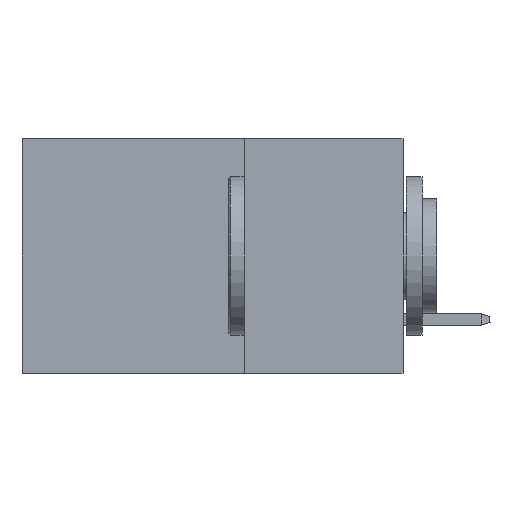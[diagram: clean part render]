
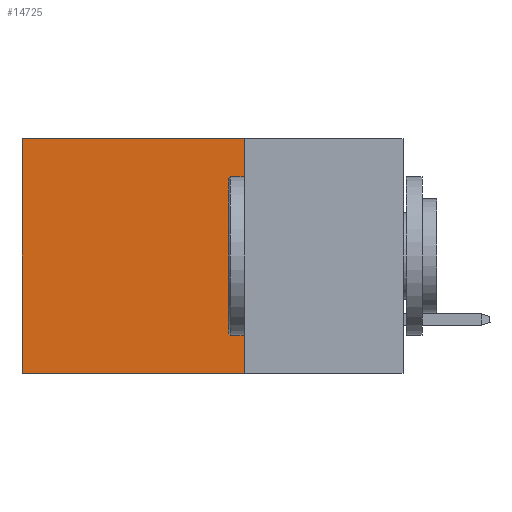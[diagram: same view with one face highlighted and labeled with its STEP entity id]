
A CAD part, left-side view. The second image highlights one B-rep face of the part: STEP entity #14725.
In plain terms, the highlighted planar face has unit normal (-1, 0, 0).
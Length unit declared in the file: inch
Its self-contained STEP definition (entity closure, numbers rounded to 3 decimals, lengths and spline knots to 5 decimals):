
#1796 = VERTEX_POINT ( 'NONE', #13453 ) ;
#2399 = DIRECTION ( 'NONE',  ( 0., 1., 0. ) ) ;
#2880 = EDGE_LOOP ( 'NONE', ( #10272, #5958, #17042, #12707 ) ) ;
#2899 = CARTESIAN_POINT ( 'NONE',  ( 0.2875, 0.25, -0.37 ) ) ;
#2921 = DIRECTION ( 'NONE',  ( 0., 1., 0. ) ) ;
#5958 = ORIENTED_EDGE ( 'NONE', *, *, #7726, .F. ) ;
#6275 = EDGE_CURVE ( 'NONE', #1796, #13255, #18011, .T. ) ;
#6816 = CARTESIAN_POINT ( 'NONE',  ( 0.2875, 0.25, 0. ) ) ;
#7195 = DIRECTION ( 'NONE',  ( 0., 0., -1. ) ) ;
#7394 = EDGE_CURVE ( 'NONE', #13255, #9412, #13055, .T. ) ;
#7621 = CARTESIAN_POINT ( 'NONE',  ( 0.2875, 0.6, 0. ) ) ;
#7726 = EDGE_CURVE ( 'NONE', #11659, #9412, #8564, .T. ) ;
#8051 = VECTOR ( 'NONE', #22057, 39.37008 ) ;
#8564 = LINE ( 'NONE', #2899, #11946 ) ;
#9412 = VERTEX_POINT ( 'NONE', #21505 ) ;
#9560 = VECTOR ( 'NONE', #7195, 39.37008 ) ;
#10272 = ORIENTED_EDGE ( 'NONE', *, *, #7394, .T. ) ;
#10912 = CARTESIAN_POINT ( 'NONE',  ( 0.2875, 0.25, 0. ) ) ;
#10919 = AXIS2_PLACEMENT_3D ( 'NONE', #10912, #16372, #24091 ) ;
#11174 = CARTESIAN_POINT ( 'NONE',  ( 0.2875, 0.6, 0. ) ) ;
#11659 = VERTEX_POINT ( 'NONE', #19801 ) ;
#11946 = VECTOR ( 'NONE', #2399, 39.37008 ) ;
#12145 = EDGE_CURVE ( 'NONE', #1796, #11659, #20292, .T. ) ;
#12707 = ORIENTED_EDGE ( 'NONE', *, *, #6275, .T. ) ;
#13055 = LINE ( 'NONE', #11174, #9560 ) ;
#13255 = VERTEX_POINT ( 'NONE', #7621 ) ;
#13453 = CARTESIAN_POINT ( 'NONE',  ( 0.2875, 0.25, 0. ) ) ;
#14725 = ADVANCED_FACE ( 'NONE', ( #20289 ), #18137, .F. ) ;
#16372 = DIRECTION ( 'NONE',  ( 1., 0., 0. ) ) ;
#17042 = ORIENTED_EDGE ( 'NONE', *, *, #12145, .F. ) ;
#18011 = LINE ( 'NONE', #20172, #22013 ) ;
#18137 = PLANE ( 'NONE',  #10919 ) ;
#19801 = CARTESIAN_POINT ( 'NONE',  ( 0.2875, 0.25, -0.37 ) ) ;
#20172 = CARTESIAN_POINT ( 'NONE',  ( 0.2875, 0.25, 0. ) ) ;
#20289 = FACE_OUTER_BOUND ( 'NONE', #2880, .T. ) ;
#20292 = LINE ( 'NONE', #6816, #8051 ) ;
#21505 = CARTESIAN_POINT ( 'NONE',  ( 0.2875, 0.6, -0.37 ) ) ;
#22013 = VECTOR ( 'NONE', #2921, 39.37008 ) ;
#22057 = DIRECTION ( 'NONE',  ( 0., 0., -1. ) ) ;
#24091 = DIRECTION ( 'NONE',  ( 0., 0., -1. ) ) ;
